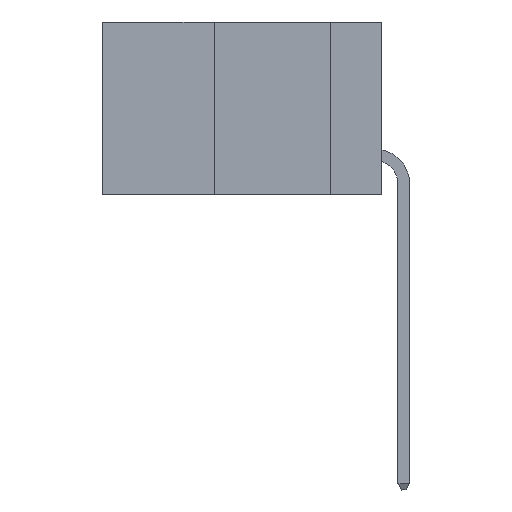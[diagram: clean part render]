
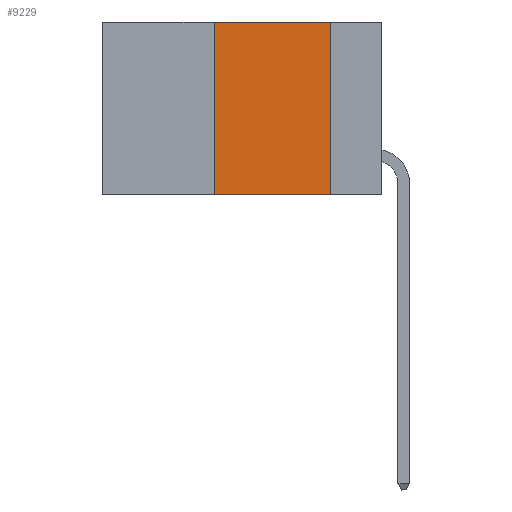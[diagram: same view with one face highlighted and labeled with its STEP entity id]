
A CAD part, left-side view. The second image highlights one B-rep face of the part: STEP entity #9229.
In plain terms, the highlighted planar face has unit normal (-1, 0, 0).
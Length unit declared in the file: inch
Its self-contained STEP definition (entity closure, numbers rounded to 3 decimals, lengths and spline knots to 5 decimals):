
#1608 = PLANE ( 'NONE',  #29066 ) ;
#1618 = EDGE_CURVE ( 'NONE', #29234, #14339, #33921, .T. ) ;
#3222 = DIRECTION ( 'NONE',  ( 0., -1., 0. ) ) ;
#8707 = ORIENTED_EDGE ( 'NONE', *, *, #10276, .F. ) ;
#9229 = ADVANCED_FACE ( 'NONE', ( #16127 ), #1608, .F. ) ;
#10276 = EDGE_CURVE ( 'NONE', #14339, #30789, #20020, .T. ) ;
#10406 = CARTESIAN_POINT ( 'NONE',  ( 0., 0.6, 0. ) ) ;
#11989 = CARTESIAN_POINT ( 'NONE',  ( 0., 0.11, -0.37 ) ) ;
#13140 = CARTESIAN_POINT ( 'NONE',  ( 0., 0.36, -0.37 ) ) ;
#14339 = VERTEX_POINT ( 'NONE', #19680 ) ;
#14693 = LINE ( 'NONE', #19886, #22362 ) ;
#14882 = CARTESIAN_POINT ( 'NONE',  ( 0., 0.6, -0.37 ) ) ;
#15775 = ORIENTED_EDGE ( 'NONE', *, *, #28847, .F. ) ;
#16127 = FACE_OUTER_BOUND ( 'NONE', #36470, .T. ) ;
#17381 = DIRECTION ( 'NONE',  ( 0., 0., -1. ) ) ;
#19680 = CARTESIAN_POINT ( 'NONE',  ( 0., 0.36, 0. ) ) ;
#19886 = CARTESIAN_POINT ( 'NONE',  ( 0., 0.11, 0. ) ) ;
#20020 = LINE ( 'NONE', #31681, #20586 ) ;
#20216 = VECTOR ( 'NONE', #30854, 39.37008 ) ;
#20586 = VECTOR ( 'NONE', #28794, 39.37008 ) ;
#20655 = LINE ( 'NONE', #14882, #21672 ) ;
#21672 = VECTOR ( 'NONE', #3222, 39.37008 ) ;
#22362 = VECTOR ( 'NONE', #17381, 39.37008 ) ;
#23217 = ORIENTED_EDGE ( 'NONE', *, *, #1618, .F. ) ;
#24193 = DIRECTION ( 'NONE',  ( 0., 0., -1. ) ) ;
#24849 = VERTEX_POINT ( 'NONE', #11989 ) ;
#25124 = CARTESIAN_POINT ( 'NONE',  ( 0., 0.36, 0. ) ) ;
#25152 = CARTESIAN_POINT ( 'NONE',  ( 0., 0.11, 0. ) ) ;
#26854 = ORIENTED_EDGE ( 'NONE', *, *, #34501, .T. ) ;
#28794 = DIRECTION ( 'NONE',  ( 0., -1., 0. ) ) ;
#28847 = EDGE_CURVE ( 'NONE', #30789, #24849, #14693, .T. ) ;
#29066 = AXIS2_PLACEMENT_3D ( 'NONE', #10406, #30089, #24193 ) ;
#29234 = VERTEX_POINT ( 'NONE', #13140 ) ;
#30089 = DIRECTION ( 'NONE',  ( 1., 0., 0. ) ) ;
#30789 = VERTEX_POINT ( 'NONE', #25152 ) ;
#30854 = DIRECTION ( 'NONE',  ( 0., 0., 1. ) ) ;
#31681 = CARTESIAN_POINT ( 'NONE',  ( 0., 0.6, 0. ) ) ;
#33921 = LINE ( 'NONE', #25124, #20216 ) ;
#34501 = EDGE_CURVE ( 'NONE', #29234, #24849, #20655, .T. ) ;
#36470 = EDGE_LOOP ( 'NONE', ( #15775, #8707, #23217, #26854 ) ) ;
